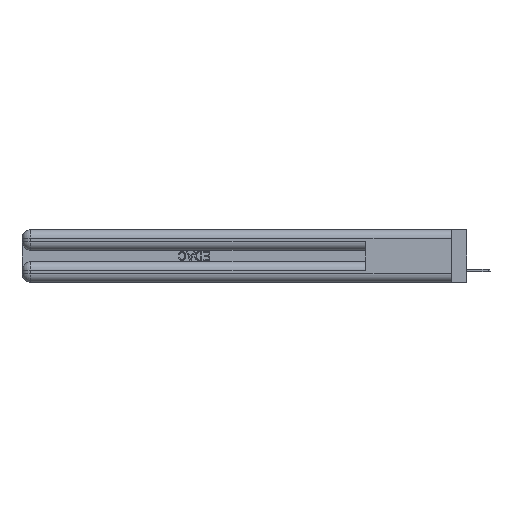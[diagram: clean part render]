
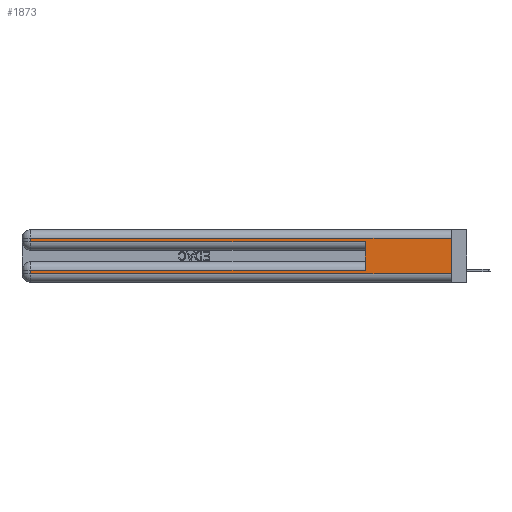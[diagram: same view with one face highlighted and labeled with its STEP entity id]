
A CAD part, left-side view. The second image highlights one B-rep face of the part: STEP entity #1873.
In plain terms, the highlighted planar face has unit normal (-1, 0, 0).
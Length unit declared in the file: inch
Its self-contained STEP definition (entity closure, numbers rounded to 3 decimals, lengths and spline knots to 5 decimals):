
#132 = VECTOR ( 'NONE', #23012, 39.37008 ) ;
#558 = VECTOR ( 'NONE', #13895, 39.37008 ) ;
#1280 = PLANE ( 'NONE',  #8939 ) ;
#1526 = CARTESIAN_POINT ( 'NONE',  ( 0., 0., 0.31 ) ) ;
#1873 = ADVANCED_FACE ( 'NONE', ( #2318 ), #1280, .F. ) ;
#2122 = CARTESIAN_POINT ( 'NONE',  ( 0., 2.94, 0.085 ) ) ;
#2318 = FACE_OUTER_BOUND ( 'NONE', #29742, .T. ) ;
#2822 = VERTEX_POINT ( 'NONE', #4866 ) ;
#3052 = VERTEX_POINT ( 'NONE', #23966 ) ;
#3220 = EDGE_CURVE ( 'NONE', #22427, #4496, #15640, .T. ) ;
#3325 = VECTOR ( 'NONE', #10105, 39.37008 ) ;
#3334 = CARTESIAN_POINT ( 'NONE',  ( 0., 0., 0.06 ) ) ;
#3495 = VERTEX_POINT ( 'NONE', #24044 ) ;
#4496 = VERTEX_POINT ( 'NONE', #3334 ) ;
#4866 = CARTESIAN_POINT ( 'NONE',  ( 0., 0.6, 0.085 ) ) ;
#6017 = VERTEX_POINT ( 'NONE', #22648 ) ;
#6439 = ORIENTED_EDGE ( 'NONE', *, *, #8640, .T. ) ;
#7837 = VECTOR ( 'NONE', #32332, 39.37008 ) ;
#8050 = CARTESIAN_POINT ( 'NONE',  ( 0., 0.6, 0.145 ) ) ;
#8640 = EDGE_CURVE ( 'NONE', #27269, #3052, #35977, .T. ) ;
#8939 = AXIS2_PLACEMENT_3D ( 'NONE', #18517, #26879, #35100 ) ;
#9808 = VECTOR ( 'NONE', #10897, 39.37008 ) ;
#10105 = DIRECTION ( 'NONE',  ( 0., 0., -1. ) ) ;
#10244 = VECTOR ( 'NONE', #34779, 39.37008 ) ;
#10897 = DIRECTION ( 'NONE',  ( 0., 0., -1. ) ) ;
#10992 = CARTESIAN_POINT ( 'NONE',  ( 0., 0., 0.285 ) ) ;
#12560 = ORIENTED_EDGE ( 'NONE', *, *, #22340, .T. ) ;
#13895 = DIRECTION ( 'NONE',  ( 0., -1., 0. ) ) ;
#14191 = EDGE_CURVE ( 'NONE', #3052, #6017, #32582, .T. ) ;
#14196 = ORIENTED_EDGE ( 'NONE', *, *, #34827, .T. ) ;
#14320 = CARTESIAN_POINT ( 'NONE',  ( 0., 2.94, 0.06 ) ) ;
#15616 = ORIENTED_EDGE ( 'NONE', *, *, #3220, .T. ) ;
#15640 = LINE ( 'NONE', #17629, #36618 ) ;
#17629 = CARTESIAN_POINT ( 'NONE',  ( 0., 0., 0.06 ) ) ;
#18517 = CARTESIAN_POINT ( 'NONE',  ( 0., 0., 0.37 ) ) ;
#18568 = EDGE_CURVE ( 'NONE', #2822, #33062, #35714, .T. ) ;
#20690 = ORIENTED_EDGE ( 'NONE', *, *, #18568, .T. ) ;
#20896 = CARTESIAN_POINT ( 'NONE',  ( 0., 0., 0.31 ) ) ;
#22340 = EDGE_CURVE ( 'NONE', #6017, #3495, #32766, .T. ) ;
#22427 = VERTEX_POINT ( 'NONE', #14320 ) ;
#22648 = CARTESIAN_POINT ( 'NONE',  ( 0., 2.94, 0.285 ) ) ;
#23012 = DIRECTION ( 'NONE',  ( 0., 0., 1. ) ) ;
#23966 = CARTESIAN_POINT ( 'NONE',  ( 0., 2.94, 0.31 ) ) ;
#24015 = CARTESIAN_POINT ( 'NONE',  ( 0., 0., 0.37 ) ) ;
#24044 = CARTESIAN_POINT ( 'NONE',  ( 0., 0.6, 0.285 ) ) ;
#25159 = CARTESIAN_POINT ( 'NONE',  ( 0., 2.94, 0.37 ) ) ;
#25679 = LINE ( 'NONE', #24015, #3325 ) ;
#26309 = CARTESIAN_POINT ( 'NONE',  ( 0., 0., 0.085 ) ) ;
#26489 = DIRECTION ( 'NONE',  ( 0., -1., 0. ) ) ;
#26505 = VECTOR ( 'NONE', #30746, 39.37008 ) ;
#26879 = DIRECTION ( 'NONE',  ( 1., 0., 0. ) ) ;
#26969 = LINE ( 'NONE', #8050, #132 ) ;
#27269 = VERTEX_POINT ( 'NONE', #1526 ) ;
#27319 = ORIENTED_EDGE ( 'NONE', *, *, #34941, .F. ) ;
#28286 = LINE ( 'NONE', #33382, #26505 ) ;
#29742 = EDGE_LOOP ( 'NONE', ( #33715, #6439, #35726, #12560, #27319, #20690, #14196, #15616 ) ) ;
#30746 = DIRECTION ( 'NONE',  ( 0., 0., -1. ) ) ;
#32332 = DIRECTION ( 'NONE',  ( 0., 1., 0. ) ) ;
#32582 = LINE ( 'NONE', #25159, #9808 ) ;
#32766 = LINE ( 'NONE', #10992, #558 ) ;
#33062 = VERTEX_POINT ( 'NONE', #2122 ) ;
#33382 = CARTESIAN_POINT ( 'NONE',  ( 0., 2.94, 0.37 ) ) ;
#33715 = ORIENTED_EDGE ( 'NONE', *, *, #33857, .F. ) ;
#33857 = EDGE_CURVE ( 'NONE', #27269, #4496, #25679, .T. ) ;
#34779 = DIRECTION ( 'NONE',  ( 0., 1., 0. ) ) ;
#34827 = EDGE_CURVE ( 'NONE', #33062, #22427, #28286, .T. ) ;
#34941 = EDGE_CURVE ( 'NONE', #2822, #3495, #26969, .T. ) ;
#35100 = DIRECTION ( 'NONE',  ( 0., 0., -1. ) ) ;
#35714 = LINE ( 'NONE', #26309, #10244 ) ;
#35726 = ORIENTED_EDGE ( 'NONE', *, *, #14191, .T. ) ;
#35977 = LINE ( 'NONE', #20896, #7837 ) ;
#36618 = VECTOR ( 'NONE', #26489, 39.37008 ) ;
